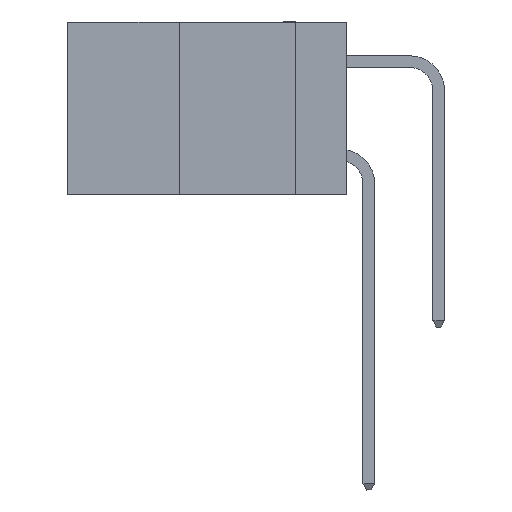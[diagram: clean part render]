
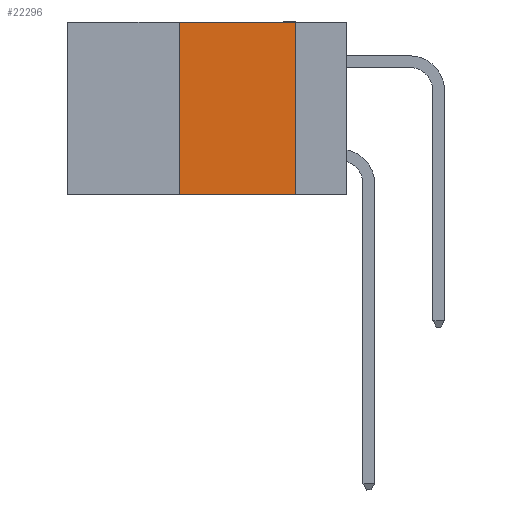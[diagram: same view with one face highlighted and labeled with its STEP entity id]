
A CAD part, left-side view. The second image highlights one B-rep face of the part: STEP entity #22296.
In plain terms, the highlighted planar face has unit normal (-1, 0, 0).
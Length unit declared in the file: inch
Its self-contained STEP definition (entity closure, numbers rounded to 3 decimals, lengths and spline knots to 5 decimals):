
#188 = DIRECTION ( 'NONE',  ( 0., 0., 1. ) ) ;
#508 = CARTESIAN_POINT ( 'NONE',  ( 0., 0.36, 0. ) ) ;
#2076 = DIRECTION ( 'NONE',  ( 1., 0., 0. ) ) ;
#2245 = VECTOR ( 'NONE', #7584, 39.37008 ) ;
#2286 = VERTEX_POINT ( 'NONE', #18871 ) ;
#2440 = ORIENTED_EDGE ( 'NONE', *, *, #12585, .T. ) ;
#4262 = VERTEX_POINT ( 'NONE', #508 ) ;
#4265 = LINE ( 'NONE', #19252, #26339 ) ;
#4905 = VERTEX_POINT ( 'NONE', #12659 ) ;
#5358 = LINE ( 'NONE', #12552, #10851 ) ;
#5907 = VECTOR ( 'NONE', #8819, 39.37008 ) ;
#7584 = DIRECTION ( 'NONE',  ( 0., 0., -1. ) ) ;
#8819 = DIRECTION ( 'NONE',  ( 0., -1., 0. ) ) ;
#10103 = VERTEX_POINT ( 'NONE', #20503 ) ;
#10157 = AXIS2_PLACEMENT_3D ( 'NONE', #16448, #2076, #16528 ) ;
#10188 = ORIENTED_EDGE ( 'NONE', *, *, #11897, .F. ) ;
#10851 = VECTOR ( 'NONE', #188, 39.37008 ) ;
#11402 = LINE ( 'NONE', #14541, #5907 ) ;
#11897 = EDGE_CURVE ( 'NONE', #4262, #10103, #11402, .T. ) ;
#12552 = CARTESIAN_POINT ( 'NONE',  ( 0., 0.36, 0. ) ) ;
#12585 = EDGE_CURVE ( 'NONE', #4905, #2286, #4265, .T. ) ;
#12659 = CARTESIAN_POINT ( 'NONE',  ( 0., 0.36, -0.37 ) ) ;
#12968 = FACE_OUTER_BOUND ( 'NONE', #22882, .T. ) ;
#14435 = PLANE ( 'NONE',  #10157 ) ;
#14541 = CARTESIAN_POINT ( 'NONE',  ( 0., 0.6, 0. ) ) ;
#16448 = CARTESIAN_POINT ( 'NONE',  ( 0., 0.6, 0. ) ) ;
#16528 = DIRECTION ( 'NONE',  ( 0., 0., -1. ) ) ;
#17161 = DIRECTION ( 'NONE',  ( 0., -1., 0. ) ) ;
#17277 = EDGE_CURVE ( 'NONE', #4905, #4262, #5358, .T. ) ;
#18596 = ORIENTED_EDGE ( 'NONE', *, *, #17277, .F. ) ;
#18740 = LINE ( 'NONE', #22052, #2245 ) ;
#18871 = CARTESIAN_POINT ( 'NONE',  ( 0., 0.11, -0.37 ) ) ;
#19252 = CARTESIAN_POINT ( 'NONE',  ( 0., 0.6, -0.37 ) ) ;
#20503 = CARTESIAN_POINT ( 'NONE',  ( 0., 0.11, 0. ) ) ;
#22052 = CARTESIAN_POINT ( 'NONE',  ( 0., 0.11, 0. ) ) ;
#22296 = ADVANCED_FACE ( 'NONE', ( #12968 ), #14435, .F. ) ;
#22882 = EDGE_LOOP ( 'NONE', ( #24515, #10188, #18596, #2440 ) ) ;
#23384 = EDGE_CURVE ( 'NONE', #10103, #2286, #18740, .T. ) ;
#24515 = ORIENTED_EDGE ( 'NONE', *, *, #23384, .F. ) ;
#26339 = VECTOR ( 'NONE', #17161, 39.37008 ) ;
